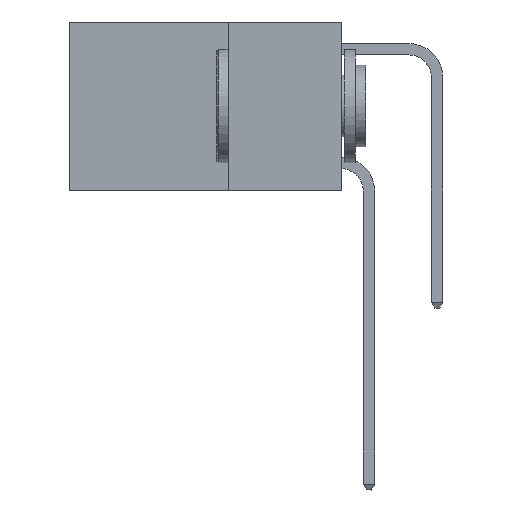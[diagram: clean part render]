
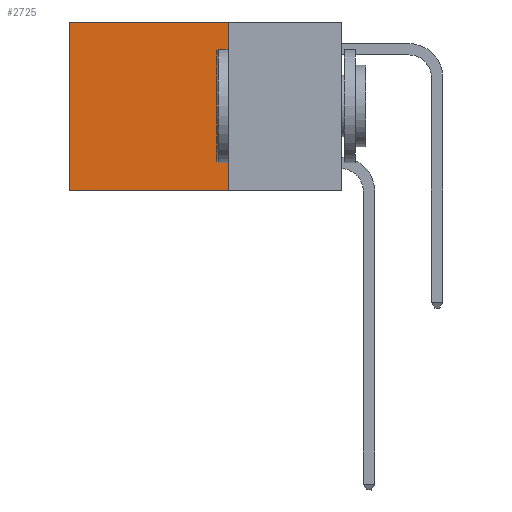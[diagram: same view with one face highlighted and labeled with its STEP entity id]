
A CAD part, left-side view. The second image highlights one B-rep face of the part: STEP entity #2725.
In plain terms, the highlighted planar face has unit normal (-1, 0, 0).
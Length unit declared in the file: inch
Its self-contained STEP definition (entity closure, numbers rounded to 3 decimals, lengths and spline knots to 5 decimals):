
#796 = CARTESIAN_POINT ( 'NONE',  ( 0.2625, 0.6, -0.37 ) ) ;
#1334 = VERTEX_POINT ( 'NONE', #10550 ) ;
#1507 = VERTEX_POINT ( 'NONE', #796 ) ;
#1566 = PLANE ( 'NONE',  #7729 ) ;
#1895 = DIRECTION ( 'NONE',  ( 0., 1., 0. ) ) ;
#2438 = EDGE_CURVE ( 'NONE', #1334, #1507, #11941, .T. ) ;
#2526 = DIRECTION ( 'NONE',  ( 1., 0., 0. ) ) ;
#2692 = CARTESIAN_POINT ( 'NONE',  ( 0.2625, 0.25, -0.37 ) ) ;
#2725 = ADVANCED_FACE ( 'NONE', ( #10433 ), #1566, .F. ) ;
#2753 = VECTOR ( 'NONE', #6209, 39.37008 ) ;
#2778 = CARTESIAN_POINT ( 'NONE',  ( 0.2625, 0.6, 0. ) ) ;
#3085 = VECTOR ( 'NONE', #1895, 39.37008 ) ;
#3481 = ORIENTED_EDGE ( 'NONE', *, *, #11918, .F. ) ;
#4228 = EDGE_CURVE ( 'NONE', #4837, #1334, #5641, .T. ) ;
#4620 = ORIENTED_EDGE ( 'NONE', *, *, #2438, .T. ) ;
#4711 = VERTEX_POINT ( 'NONE', #10685 ) ;
#4837 = VERTEX_POINT ( 'NONE', #5570 ) ;
#5570 = CARTESIAN_POINT ( 'NONE',  ( 0.2625, 0.25, 0. ) ) ;
#5641 = LINE ( 'NONE', #9315, #9185 ) ;
#5723 = DIRECTION ( 'NONE',  ( 0., 0., -1. ) ) ;
#5761 = EDGE_LOOP ( 'NONE', ( #4620, #9939, #3481, #5773 ) ) ;
#5773 = ORIENTED_EDGE ( 'NONE', *, *, #4228, .T. ) ;
#6209 = DIRECTION ( 'NONE',  ( 0., 0., -1. ) ) ;
#7729 = AXIS2_PLACEMENT_3D ( 'NONE', #8279, #2526, #9186 ) ;
#8180 = LINE ( 'NONE', #2692, #3085 ) ;
#8279 = CARTESIAN_POINT ( 'NONE',  ( 0.2625, 0.25, 0. ) ) ;
#9117 = VECTOR ( 'NONE', #5723, 39.37008 ) ;
#9185 = VECTOR ( 'NONE', #10291, 39.37008 ) ;
#9186 = DIRECTION ( 'NONE',  ( 0., 0., -1. ) ) ;
#9315 = CARTESIAN_POINT ( 'NONE',  ( 0.2625, 0.25, 0. ) ) ;
#9939 = ORIENTED_EDGE ( 'NONE', *, *, #10640, .F. ) ;
#10291 = DIRECTION ( 'NONE',  ( 0., 1., 0. ) ) ;
#10433 = FACE_OUTER_BOUND ( 'NONE', #5761, .T. ) ;
#10550 = CARTESIAN_POINT ( 'NONE',  ( 0.2625, 0.6, 0. ) ) ;
#10640 = EDGE_CURVE ( 'NONE', #4711, #1507, #8180, .T. ) ;
#10685 = CARTESIAN_POINT ( 'NONE',  ( 0.2625, 0.25, -0.37 ) ) ;
#10932 = CARTESIAN_POINT ( 'NONE',  ( 0.2625, 0.25, 0. ) ) ;
#11088 = LINE ( 'NONE', #10932, #2753 ) ;
#11918 = EDGE_CURVE ( 'NONE', #4837, #4711, #11088, .T. ) ;
#11941 = LINE ( 'NONE', #2778, #9117 ) ;
